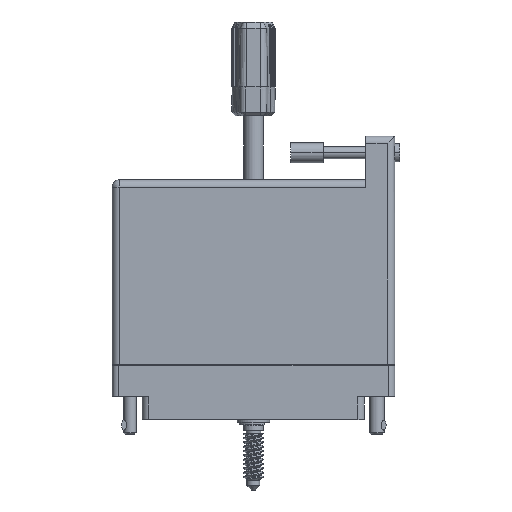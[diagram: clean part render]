
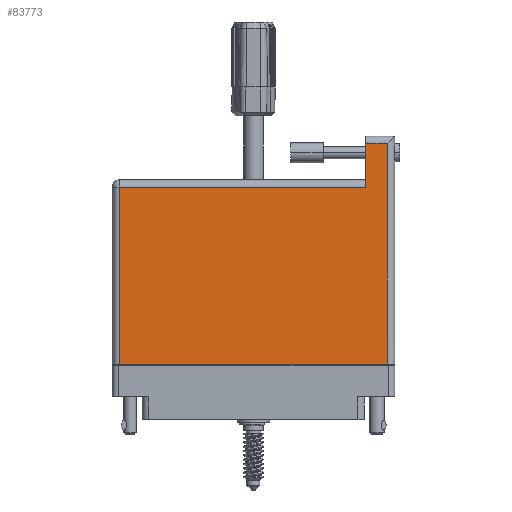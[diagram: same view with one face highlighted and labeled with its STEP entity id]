
A CAD part, front view. The second image highlights one B-rep face of the part: STEP entity #83773.
In plain terms, the highlighted face is planar.
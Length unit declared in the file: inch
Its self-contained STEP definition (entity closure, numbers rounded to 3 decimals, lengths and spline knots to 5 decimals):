
#3037 = LINE ( 'NONE', #62084, #75645 ) ;
#5128 = LINE ( 'NONE', #90927, #18303 ) ;
#10098 = ORIENTED_EDGE ( 'NONE', *, *, #20066, .T. ) ;
#14991 = PLANE ( 'NONE',  #67212 ) ;
#18303 = VECTOR ( 'NONE', #83812, 39.37008 ) ;
#19053 = CARTESIAN_POINT ( 'NONE',  ( 1.289, 2.025, 0.617 ) ) ;
#19856 = CARTESIAN_POINT ( 'NONE',  ( 1.289, 2.095, 0.617 ) ) ;
#20066 = EDGE_CURVE ( 'NONE', #69237, #40785, #5128, .T. ) ;
#20469 = DIRECTION ( 'NONE',  ( 0., 1., 0. ) ) ;
#22315 = EDGE_CURVE ( 'NONE', #34690, #69237, #87222, .T. ) ;
#23068 = FACE_OUTER_BOUND ( 'NONE', #71334, .T. ) ;
#29123 = DIRECTION ( 'NONE',  ( -1., 0., 0. ) ) ;
#30053 = CARTESIAN_POINT ( 'NONE',  ( -1.359, 1.675, 0.617 ) ) ;
#30069 = LINE ( 'NONE', #31828, #44400 ) ;
#30731 = VECTOR ( 'NONE', #78506, 39.37008 ) ;
#31828 = CARTESIAN_POINT ( 'NONE',  ( -1.359, 2.025, 0.617 ) ) ;
#32736 = CARTESIAN_POINT ( 'NONE',  ( -1.289, -0.1, 0.617 ) ) ;
#34690 = VERTEX_POINT ( 'NONE', #81698 ) ;
#39031 = EDGE_CURVE ( 'NONE', #40785, #56571, #3037, .T. ) ;
#40123 = EDGE_CURVE ( 'NONE', #56571, #59005, #57189, .T. ) ;
#40785 = VERTEX_POINT ( 'NONE', #87394 ) ;
#43510 = CARTESIAN_POINT ( 'NONE',  ( -1.359, -0.1, 0.617 ) ) ;
#44400 = VECTOR ( 'NONE', #88073, 39.37008 ) ;
#47671 = DIRECTION ( 'NONE',  ( 0., -1., 0. ) ) ;
#48758 = DIRECTION ( 'NONE',  ( 0., -1., 0. ) ) ;
#48826 = ORIENTED_EDGE ( 'NONE', *, *, #61975, .T. ) ;
#53422 = ORIENTED_EDGE ( 'NONE', *, *, #87073, .T. ) ;
#53808 = ORIENTED_EDGE ( 'NONE', *, *, #39031, .T. ) ;
#56571 = VERTEX_POINT ( 'NONE', #32736 ) ;
#56832 = ORIENTED_EDGE ( 'NONE', *, *, #22315, .T. ) ;
#57189 = LINE ( 'NONE', #43510, #30731 ) ;
#59005 = VERTEX_POINT ( 'NONE', #63430 ) ;
#61975 = EDGE_CURVE ( 'NONE', #59005, #80120, #80023, .T. ) ;
#62084 = CARTESIAN_POINT ( 'NONE',  ( -1.289, -0.1, 0.617 ) ) ;
#63430 = CARTESIAN_POINT ( 'NONE',  ( 1.289, -0.1, 0.617 ) ) ;
#63528 = VECTOR ( 'NONE', #20469, 39.37008 ) ;
#67212 = AXIS2_PLACEMENT_3D ( 'NONE', #30053, #85034, #29123 ) ;
#68580 = VECTOR ( 'NONE', #48758, 39.37008 ) ;
#69237 = VERTEX_POINT ( 'NONE', #84857 ) ;
#69977 = CARTESIAN_POINT ( 'NONE',  ( 1.079, 2.095, 0.617 ) ) ;
#71334 = EDGE_LOOP ( 'NONE', ( #10098, #53808, #72349, #48826, #53422, #56832 ) ) ;
#72349 = ORIENTED_EDGE ( 'NONE', *, *, #40123, .T. ) ;
#75645 = VECTOR ( 'NONE', #47671, 39.37008 ) ;
#78506 = DIRECTION ( 'NONE',  ( 1., 0., 0. ) ) ;
#80023 = LINE ( 'NONE', #19856, #63528 ) ;
#80120 = VERTEX_POINT ( 'NONE', #19053 ) ;
#81698 = CARTESIAN_POINT ( 'NONE',  ( 1.079, 2.025, 0.617 ) ) ;
#83773 = ADVANCED_FACE ( 'NONE', ( #23068 ), #14991, .F. ) ;
#83812 = DIRECTION ( 'NONE',  ( -1., 0., 0. ) ) ;
#84857 = CARTESIAN_POINT ( 'NONE',  ( 1.079, 1.605, 0.617 ) ) ;
#85034 = DIRECTION ( 'NONE',  ( 0., 0., -1. ) ) ;
#87073 = EDGE_CURVE ( 'NONE', #80120, #34690, #30069, .T. ) ;
#87222 = LINE ( 'NONE', #69977, #68580 ) ;
#87394 = CARTESIAN_POINT ( 'NONE',  ( -1.289, 1.605, 0.617 ) ) ;
#88073 = DIRECTION ( 'NONE',  ( -1., 0., 0. ) ) ;
#90927 = CARTESIAN_POINT ( 'NONE',  ( -1.359, 1.605, 0.617 ) ) ;
